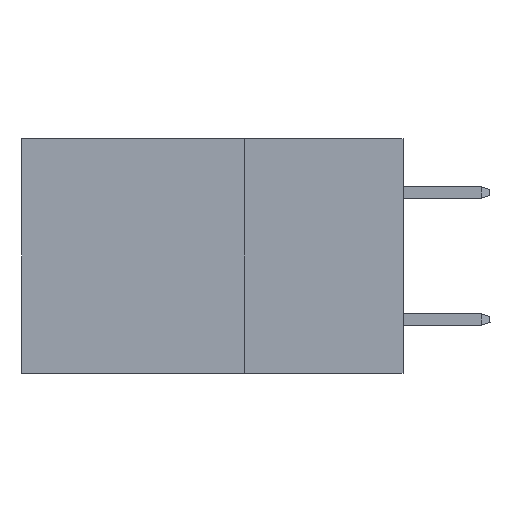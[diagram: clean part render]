
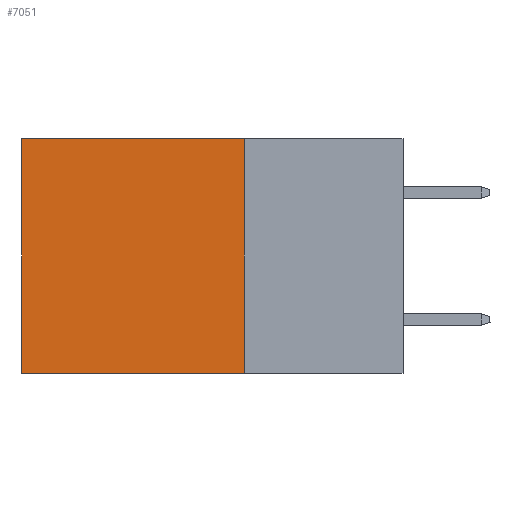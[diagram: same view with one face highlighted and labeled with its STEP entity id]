
A CAD part, left-side view. The second image highlights one B-rep face of the part: STEP entity #7051.
In plain terms, the highlighted planar face has unit normal (-1, 0, 0).
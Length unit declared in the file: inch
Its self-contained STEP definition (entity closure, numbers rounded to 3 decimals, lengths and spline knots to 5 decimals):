
#935 = EDGE_CURVE ( 'NONE', #15434, #1099, #18234, .T. ) ;
#1099 = VERTEX_POINT ( 'NONE', #12251 ) ;
#1519 = CARTESIAN_POINT ( 'NONE',  ( 0.2875, 0.25, 0. ) ) ;
#1780 = CARTESIAN_POINT ( 'NONE',  ( 0.2875, 0.25, -0.37 ) ) ;
#2258 = CARTESIAN_POINT ( 'NONE',  ( 0.2875, 0.25, 0. ) ) ;
#2415 = CARTESIAN_POINT ( 'NONE',  ( 0.2875, 0.6, 0. ) ) ;
#2628 = EDGE_CURVE ( 'NONE', #10897, #20445, #7789, .T. ) ;
#3002 = VECTOR ( 'NONE', #16723, 39.37008 ) ;
#4880 = VECTOR ( 'NONE', #11160, 39.37008 ) ;
#4902 = EDGE_CURVE ( 'NONE', #20445, #1099, #13038, .T. ) ;
#5779 = CARTESIAN_POINT ( 'NONE',  ( 0.2875, 0.25, 0. ) ) ;
#6020 = CARTESIAN_POINT ( 'NONE',  ( 0.2875, 0.25, 0. ) ) ;
#6250 = ORIENTED_EDGE ( 'NONE', *, *, #2628, .F. ) ;
#7051 = ADVANCED_FACE ( 'NONE', ( #19249 ), #11869, .F. ) ;
#7789 = LINE ( 'NONE', #6020, #4880 ) ;
#9289 = LINE ( 'NONE', #5779, #20901 ) ;
#10897 = VERTEX_POINT ( 'NONE', #2258 ) ;
#11160 = DIRECTION ( 'NONE',  ( 0., 0., -1. ) ) ;
#11382 = DIRECTION ( 'NONE',  ( 0., 1., 0. ) ) ;
#11869 = PLANE ( 'NONE',  #19403 ) ;
#12251 = CARTESIAN_POINT ( 'NONE',  ( 0.2875, 0.6, -0.37 ) ) ;
#12417 = EDGE_LOOP ( 'NONE', ( #12697, #18488, #6250, #17644 ) ) ;
#12585 = EDGE_CURVE ( 'NONE', #10897, #15434, #9289, .T. ) ;
#12697 = ORIENTED_EDGE ( 'NONE', *, *, #935, .T. ) ;
#13038 = LINE ( 'NONE', #21838, #18778 ) ;
#13988 = DIRECTION ( 'NONE',  ( 1., 0., 0. ) ) ;
#14102 = DIRECTION ( 'NONE',  ( 0., 0., -1. ) ) ;
#15434 = VERTEX_POINT ( 'NONE', #18308 ) ;
#16723 = DIRECTION ( 'NONE',  ( 0., 0., -1. ) ) ;
#17644 = ORIENTED_EDGE ( 'NONE', *, *, #12585, .T. ) ;
#18234 = LINE ( 'NONE', #2415, #3002 ) ;
#18308 = CARTESIAN_POINT ( 'NONE',  ( 0.2875, 0.6, 0. ) ) ;
#18488 = ORIENTED_EDGE ( 'NONE', *, *, #4902, .F. ) ;
#18778 = VECTOR ( 'NONE', #20074, 39.37008 ) ;
#19249 = FACE_OUTER_BOUND ( 'NONE', #12417, .T. ) ;
#19403 = AXIS2_PLACEMENT_3D ( 'NONE', #1519, #13988, #14102 ) ;
#20074 = DIRECTION ( 'NONE',  ( 0., 1., 0. ) ) ;
#20445 = VERTEX_POINT ( 'NONE', #1780 ) ;
#20901 = VECTOR ( 'NONE', #11382, 39.37008 ) ;
#21838 = CARTESIAN_POINT ( 'NONE',  ( 0.2875, 0.25, -0.37 ) ) ;
